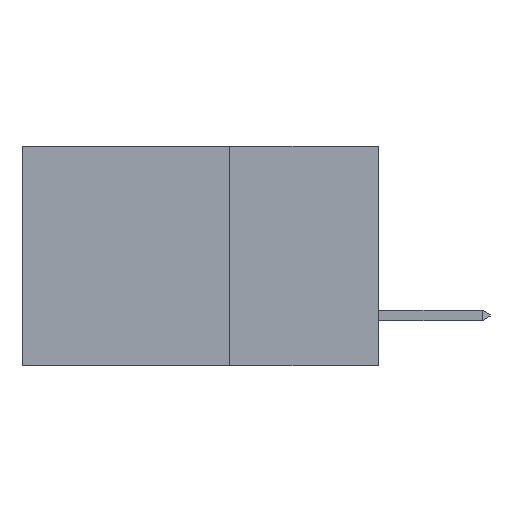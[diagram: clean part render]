
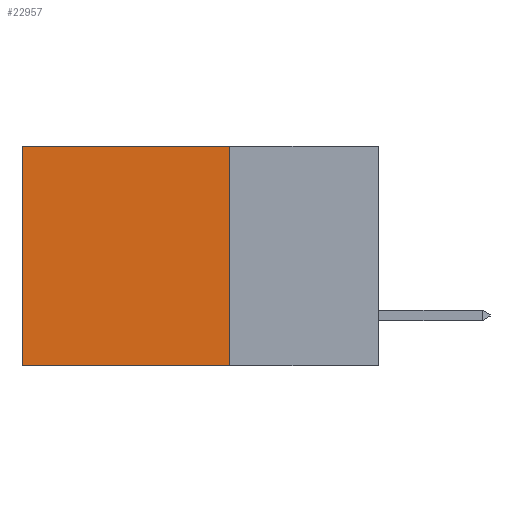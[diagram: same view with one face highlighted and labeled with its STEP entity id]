
A CAD part, left-side view. The second image highlights one B-rep face of the part: STEP entity #22957.
In plain terms, the highlighted planar face has unit normal (-1, 0, 0).
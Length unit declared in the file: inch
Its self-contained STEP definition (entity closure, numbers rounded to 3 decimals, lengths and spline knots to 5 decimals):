
#1774 = EDGE_LOOP ( 'NONE', ( #18286, #4290, #3242, #5508 ) ) ;
#2481 = CARTESIAN_POINT ( 'NONE',  ( 0.298, 0.25, 0. ) ) ;
#3242 = ORIENTED_EDGE ( 'NONE', *, *, #8959, .F. ) ;
#3905 = PLANE ( 'NONE',  #8160 ) ;
#3969 = VERTEX_POINT ( 'NONE', #16797 ) ;
#4290 = ORIENTED_EDGE ( 'NONE', *, *, #8884, .F. ) ;
#5508 = ORIENTED_EDGE ( 'NONE', *, *, #18618, .T. ) ;
#5876 = VERTEX_POINT ( 'NONE', #26706 ) ;
#7886 = CARTESIAN_POINT ( 'NONE',  ( 0.298, 0.6, 0. ) ) ;
#8137 = LINE ( 'NONE', #20043, #13508 ) ;
#8160 = AXIS2_PLACEMENT_3D ( 'NONE', #19894, #22128, #8542 ) ;
#8313 = FACE_OUTER_BOUND ( 'NONE', #1774, .T. ) ;
#8542 = DIRECTION ( 'NONE',  ( 0., 0., -1. ) ) ;
#8707 = DIRECTION ( 'NONE',  ( 0., 1., 0. ) ) ;
#8884 = EDGE_CURVE ( 'NONE', #5876, #15964, #8137, .T. ) ;
#8959 = EDGE_CURVE ( 'NONE', #3969, #5876, #24110, .T. ) ;
#9441 = DIRECTION ( 'NONE',  ( 0., 1., 0. ) ) ;
#10207 = DIRECTION ( 'NONE',  ( 0., 0., -1. ) ) ;
#10299 = CARTESIAN_POINT ( 'NONE',  ( 0.298, 0.6, -0.37 ) ) ;
#13508 = VECTOR ( 'NONE', #8707, 39.37008 ) ;
#15925 = EDGE_CURVE ( 'NONE', #18129, #15964, #29240, .T. ) ;
#15964 = VERTEX_POINT ( 'NONE', #10299 ) ;
#16797 = CARTESIAN_POINT ( 'NONE',  ( 0.298, 0.25, 0. ) ) ;
#18129 = VERTEX_POINT ( 'NONE', #20868 ) ;
#18286 = ORIENTED_EDGE ( 'NONE', *, *, #15925, .T. ) ;
#18618 = EDGE_CURVE ( 'NONE', #3969, #18129, #25286, .T. ) ;
#19337 = VECTOR ( 'NONE', #9441, 39.37008 ) ;
#19894 = CARTESIAN_POINT ( 'NONE',  ( 0.298, 0.25, 0. ) ) ;
#20043 = CARTESIAN_POINT ( 'NONE',  ( 0.298, 0.25, -0.37 ) ) ;
#20868 = CARTESIAN_POINT ( 'NONE',  ( 0.298, 0.6, 0. ) ) ;
#22128 = DIRECTION ( 'NONE',  ( 1., 0., 0. ) ) ;
#22499 = CARTESIAN_POINT ( 'NONE',  ( 0.298, 0.25, 0. ) ) ;
#22957 = ADVANCED_FACE ( 'NONE', ( #8313 ), #3905, .F. ) ;
#23413 = VECTOR ( 'NONE', #29211, 39.37008 ) ;
#24110 = LINE ( 'NONE', #22499, #23413 ) ;
#25286 = LINE ( 'NONE', #2481, #19337 ) ;
#25430 = VECTOR ( 'NONE', #10207, 39.37008 ) ;
#26706 = CARTESIAN_POINT ( 'NONE',  ( 0.298, 0.25, -0.37 ) ) ;
#29211 = DIRECTION ( 'NONE',  ( 0., 0., -1. ) ) ;
#29240 = LINE ( 'NONE', #7886, #25430 ) ;
